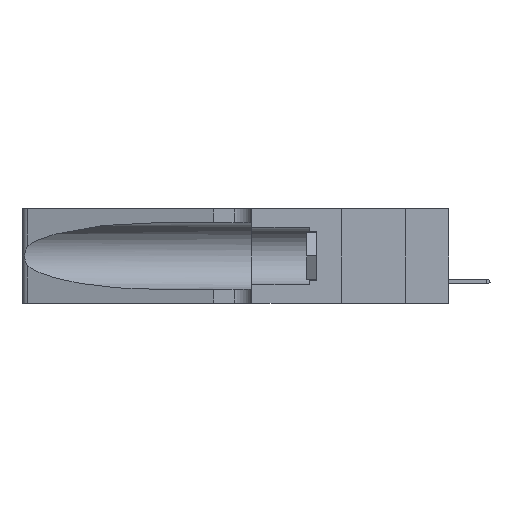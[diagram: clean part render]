
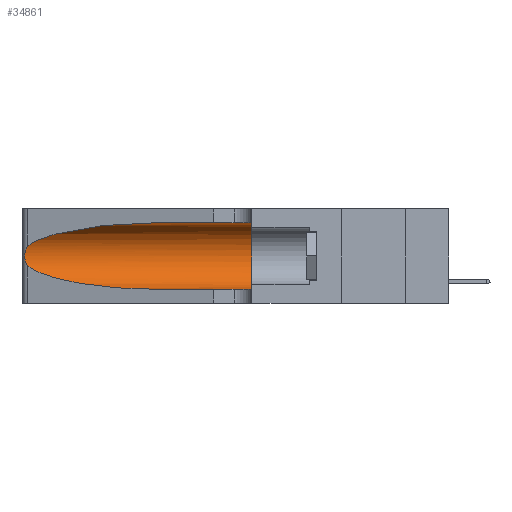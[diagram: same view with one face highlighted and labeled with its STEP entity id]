
A CAD part, left-side view. The second image highlights one B-rep face of the part: STEP entity #34861.
In plain terms, the highlighted cylindrical face has radius 3.308 mm (diameter 6.617 mm), a partial arc.
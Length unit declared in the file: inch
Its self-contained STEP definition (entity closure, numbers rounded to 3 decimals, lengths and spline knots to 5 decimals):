
#3553 = VERTEX_POINT ( 'NONE', #18910 ) ;
#3895 =( BOUNDED_CURVE ( )  B_SPLINE_CURVE ( 3, ( #8411, #41181, #45599, #37227 ),
 .UNSPECIFIED., .F., .F. ) 
 B_SPLINE_CURVE_WITH_KNOTS ( ( 4, 4 ),
 ( 3.44316, 4.71239 ),
 .UNSPECIFIED. ) 
 CURVE ( )  GEOMETRIC_REPRESENTATION_ITEM ( )  RATIONAL_B_SPLINE_CURVE ( ( 1., 0.87, 0.87, 1. ) ) 
 REPRESENTATION_ITEM ( '' )  );
#4359 = EDGE_CURVE ( 'NONE', #4479, #9348, #32956, .T. ) ;
#4479 = VERTEX_POINT ( 'NONE', #40371 ) ;
#4903 = CARTESIAN_POINT ( 'NONE',  ( 0.1305, 1.61858, 0.31525 ) ) ;
#5009 = CARTESIAN_POINT ( 'NONE',  ( 0.25639, 1.23186, 0.15144 ) ) ;
#5687 = CARTESIAN_POINT ( 'NONE',  ( 0.2373, 1.15595, 0.28018 ) ) ;
#5715 = CARTESIAN_POINT ( 'NONE',  ( 0.25789, 1.23486, 0.15765 ) ) ;
#6491 = VERTEX_POINT ( 'NONE', #50474 ) ;
#7382 = DIRECTION ( 'NONE',  ( 0., 0., 1. ) ) ;
#8411 = CARTESIAN_POINT ( 'NONE',  ( 0.25487, 1.22718, 0.14631 ) ) ;
#8415 =( BOUNDED_CURVE ( )  B_SPLINE_CURVE ( 3, ( #29732, #46118, #5687, #13449 ),
 .UNSPECIFIED., .F., .F. ) 
 B_SPLINE_CURVE_WITH_KNOTS ( ( 4, 4 ),
 ( 1.5708, 2.84003 ),
 .UNSPECIFIED. ) 
 CURVE ( )  GEOMETRIC_REPRESENTATION_ITEM ( )  RATIONAL_B_SPLINE_CURVE ( ( 1., 0.87, 0.87, 1. ) ) 
 REPRESENTATION_ITEM ( '' )  );
#9348 = VERTEX_POINT ( 'NONE', #39396 ) ;
#9469 = EDGE_CURVE ( 'NONE', #6491, #23041, #42340, .T. ) ;
#10352 = ORIENTED_EDGE ( 'NONE', *, *, #9469, .T. ) ;
#12532 = EDGE_CURVE ( 'NONE', #9348, #23041, #34904, .T. ) ;
#13068 = VECTOR ( 'NONE', #18359, 39.37008 ) ;
#13449 = CARTESIAN_POINT ( 'NONE',  ( 0.25487, 1.22718, 0.22369 ) ) ;
#14242 = CARTESIAN_POINT ( 'NONE',  ( 0.1305, 1.61858, 0.05475 ) ) ;
#15371 = CARTESIAN_POINT ( 'NONE',  ( 0.1305, 0.35, 0.185 ) ) ;
#17767 = CARTESIAN_POINT ( 'NONE',  ( 0.25487, 1.22718, 0.14631 ) ) ;
#18359 = DIRECTION ( 'NONE',  ( 0., -1., 0. ) ) ;
#18414 = CARTESIAN_POINT ( 'NONE',  ( 0.1305, 0.35, 0.05475 ) ) ;
#18910 = CARTESIAN_POINT ( 'NONE',  ( 0.25487, 1.22718, 0.22369 ) ) ;
#19151 = ORIENTED_EDGE ( 'NONE', *, *, #23591, .T. ) ;
#21823 = CARTESIAN_POINT ( 'NONE',  ( 0.25854, 1.2359, 0.20912 ) ) ;
#23041 = VERTEX_POINT ( 'NONE', #18414 ) ;
#23591 = EDGE_CURVE ( 'NONE', #3553, #34136, #38237, .T. ) ;
#23954 = EDGE_CURVE ( 'NONE', #34136, #6491, #3895, .T. ) ;
#24927 = CARTESIAN_POINT ( 'NONE',  ( 0.1305, 1.61858, 0.185 ) ) ;
#27886 = DIRECTION ( 'NONE',  ( 0., 1., 0. ) ) ;
#29732 = CARTESIAN_POINT ( 'NONE',  ( 0.1305, 0.72297, 0.31525 ) ) ;
#31067 = EDGE_CURVE ( 'NONE', #4479, #3553, #8415, .T. ) ;
#31129 = DIRECTION ( 'NONE',  ( 0., -1., 0. ) ) ;
#32127 = ORIENTED_EDGE ( 'NONE', *, *, #31067, .T. ) ;
#32397 = ORIENTED_EDGE ( 'NONE', *, *, #4359, .F. ) ;
#32956 = LINE ( 'NONE', #4903, #37390 ) ;
#33310 = CARTESIAN_POINT ( 'NONE',  ( 0.25555, 1.22993, 0.14849 ) ) ;
#33322 = CARTESIAN_POINT ( 'NONE',  ( 0.26075, 1.23896, 0.19203 ) ) ;
#34136 = VERTEX_POINT ( 'NONE', #40165 ) ;
#34861 = ADVANCED_FACE ( 'NONE', ( #35744 ), #45215, .F. ) ;
#34904 = CIRCLE ( 'NONE', #45832, 0.13025 ) ;
#35025 = EDGE_LOOP ( 'NONE', ( #32127, #19151, #48274, #10352, #37463, #32397 ) ) ;
#35744 = FACE_OUTER_BOUND ( 'NONE', #35025, .T. ) ;
#35951 = DIRECTION ( 'NONE',  ( 0., 0., -1. ) ) ;
#37227 = CARTESIAN_POINT ( 'NONE',  ( 0.1305, 0.72297, 0.05475 ) ) ;
#37390 = VECTOR ( 'NONE', #42480, 39.37008 ) ;
#37463 = ORIENTED_EDGE ( 'NONE', *, *, #12532, .F. ) ;
#38237 = B_SPLINE_CURVE_WITH_KNOTS ( 'NONE', 3,
 ( #51441, #39358, #52434, #48840, #21823, #43627, #33322, #44501, #41526, #42046, #5715, #5009, #33310, #17767 ),
 .UNSPECIFIED., .F., .F.,
 ( 4, 2, 2, 2, 2, 2, 4 ),
 ( 0., 0.00027, 0.00053, 0.00107, 0.0016, 0.00187, 0.00214 ),
 .UNSPECIFIED. ) ;
#39358 = CARTESIAN_POINT ( 'NONE',  ( 0.25555, 1.22994, 0.2215 ) ) ;
#39396 = CARTESIAN_POINT ( 'NONE',  ( 0.1305, 0.35, 0.31525 ) ) ;
#40165 = CARTESIAN_POINT ( 'NONE',  ( 0.25487, 1.22718, 0.14631 ) ) ;
#40371 = CARTESIAN_POINT ( 'NONE',  ( 0.1305, 0.72297, 0.31525 ) ) ;
#41181 = CARTESIAN_POINT ( 'NONE',  ( 0.2373, 1.15595, 0.08982 ) ) ;
#41526 = CARTESIAN_POINT ( 'NONE',  ( 0.26017, 1.23833, 0.17102 ) ) ;
#42046 = CARTESIAN_POINT ( 'NONE',  ( 0.25856, 1.23593, 0.16098 ) ) ;
#42340 = LINE ( 'NONE', #14242, #13068 ) ;
#42480 = DIRECTION ( 'NONE',  ( 0., -1., 0. ) ) ;
#43627 = CARTESIAN_POINT ( 'NONE',  ( 0.26018, 1.23835, 0.19895 ) ) ;
#44501 = CARTESIAN_POINT ( 'NONE',  ( 0.26075, 1.23896, 0.178 ) ) ;
#44886 = AXIS2_PLACEMENT_3D ( 'NONE', #24927, #31129, #35951 ) ;
#45215 = CYLINDRICAL_SURFACE ( 'NONE', #44886, 0.13025 ) ;
#45599 = CARTESIAN_POINT ( 'NONE',  ( 0.18966, 0.96281, 0.05475 ) ) ;
#45832 = AXIS2_PLACEMENT_3D ( 'NONE', #15371, #27886, #7382 ) ;
#46118 = CARTESIAN_POINT ( 'NONE',  ( 0.18966, 0.96281, 0.31525 ) ) ;
#48274 = ORIENTED_EDGE ( 'NONE', *, *, #23954, .T. ) ;
#48840 = CARTESIAN_POINT ( 'NONE',  ( 0.25787, 1.23484, 0.2124 ) ) ;
#50474 = CARTESIAN_POINT ( 'NONE',  ( 0.1305, 0.72297, 0.05475 ) ) ;
#51441 = CARTESIAN_POINT ( 'NONE',  ( 0.25487, 1.22718, 0.22369 ) ) ;
#52434 = CARTESIAN_POINT ( 'NONE',  ( 0.25639, 1.23184, 0.21858 ) ) ;
